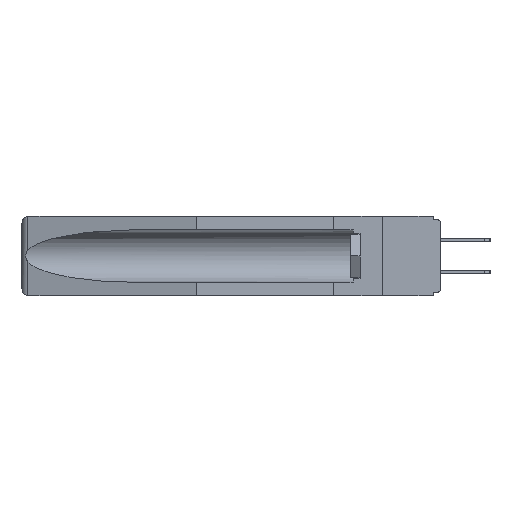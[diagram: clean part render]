
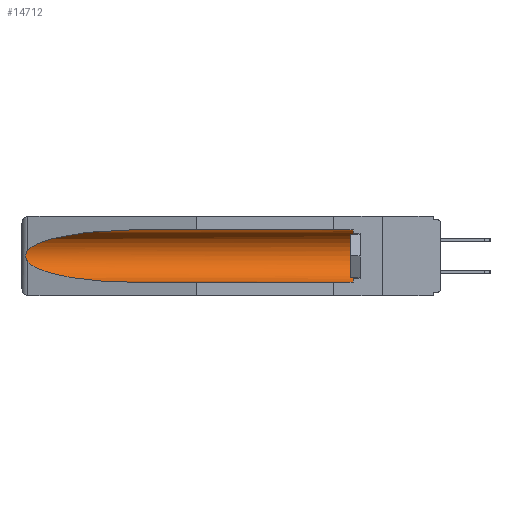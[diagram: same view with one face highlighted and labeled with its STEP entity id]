
A CAD part, left-side view. The second image highlights one B-rep face of the part: STEP entity #14712.
In plain terms, the highlighted cylindrical face has radius 2.857 mm (diameter 5.715 mm), a partial arc.
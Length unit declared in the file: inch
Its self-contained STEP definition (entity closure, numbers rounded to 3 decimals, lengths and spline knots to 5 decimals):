
#1440 = CARTESIAN_POINT ( 'NONE',  ( 0.26654, 1.53092, -0.15636 ) ) ;
#1944 = CARTESIAN_POINT ( 'NONE',  ( 0.155, 0.126, -0.1715 ) ) ;
#2196 = EDGE_CURVE ( 'NONE', #29372, #29384, #31087, .T. ) ;
#2393 = CARTESIAN_POINT ( 'NONE',  ( 0.155, 1.07973, -0.059 ) ) ;
#2695 = LINE ( 'NONE', #21639, #15614 ) ;
#3336 = EDGE_LOOP ( 'NONE', ( #25295, #10266, #11486, #13064, #22401, #14451 ) ) ;
#3780 =( BOUNDED_CURVE ( )  B_SPLINE_CURVE ( 3, ( #4491, #21707, #9361, #7116 ),
 .UNSPECIFIED., .F., .F. ) 
 B_SPLINE_CURVE_WITH_KNOTS ( ( 4, 4 ),
 ( 0.1948, 1.5708 ),
 .UNSPECIFIED. ) 
 CURVE ( )  GEOMETRIC_REPRESENTATION_ITEM ( )  RATIONAL_B_SPLINE_CURVE ( ( 1., 0.848, 0.848, 1. ) ) 
 REPRESENTATION_ITEM ( '' )  );
#3962 = VECTOR ( 'NONE', #27473, 39.37008 ) ;
#4127 = DIRECTION ( 'NONE',  ( 0., 1., 0. ) ) ;
#4421 = CARTESIAN_POINT ( 'NONE',  ( 0.26655, 1.53094, -0.18657 ) ) ;
#4491 = CARTESIAN_POINT ( 'NONE',  ( 0.26537, 1.52718, -0.19328 ) ) ;
#4747 = CARTESIAN_POINT ( 'NONE',  ( 0.2673, 1.53269, -0.17917 ) ) ;
#4952 = CARTESIAN_POINT ( 'NONE',  ( 0.25451, 1.48313, -0.09465 ) ) ;
#6329 = CARTESIAN_POINT ( 'NONE',  ( 0.26537, 1.52718, -0.14972 ) ) ;
#7116 = CARTESIAN_POINT ( 'NONE',  ( 0.155, 1.07973, -0.284 ) ) ;
#7553 = EDGE_CURVE ( 'NONE', #14687, #25336, #3780, .T. ) ;
#8666 = EDGE_CURVE ( 'NONE', #29384, #24623, #2695, .T. ) ;
#9361 = CARTESIAN_POINT ( 'NONE',  ( 0.21114, 1.30732, -0.284 ) ) ;
#9494 = CARTESIAN_POINT ( 'NONE',  ( 0.26537, 1.52718, -0.14972 ) ) ;
#9511 = CARTESIAN_POINT ( 'NONE',  ( 0.2675, 1.53308, -0.17534 ) ) ;
#10046 = LINE ( 'NONE', #15360, #3962 ) ;
#10266 = ORIENTED_EDGE ( 'NONE', *, *, #24511, .T. ) ;
#11486 = ORIENTED_EDGE ( 'NONE', *, *, #7553, .T. ) ;
#11538 = CARTESIAN_POINT ( 'NONE',  ( 0.26537, 1.52718, -0.19328 ) ) ;
#12795 = EDGE_CURVE ( 'NONE', #29372, #25336, #10046, .T. ) ;
#13064 = ORIENTED_EDGE ( 'NONE', *, *, #12795, .F. ) ;
#13914 = AXIS2_PLACEMENT_3D ( 'NONE', #1944, #19039, #16716 ) ;
#14169 = CARTESIAN_POINT ( 'NONE',  ( 0.2675, 1.53308, -0.16763 ) ) ;
#14294 = CARTESIAN_POINT ( 'NONE',  ( 0.155, -0.30754, -0.1715 ) ) ;
#14451 = ORIENTED_EDGE ( 'NONE', *, *, #8666, .T. ) ;
#14687 = VERTEX_POINT ( 'NONE', #11538 ) ;
#14712 = ADVANCED_FACE ( 'NONE', ( #22601 ), #14773, .F. ) ;
#14773 = CYLINDRICAL_SURFACE ( 'NONE', #18576, 0.1125 ) ;
#15360 = CARTESIAN_POINT ( 'NONE',  ( 0.155, -0.30754, -0.284 ) ) ;
#15436 = VERTEX_POINT ( 'NONE', #9494 ) ;
#15614 = VECTOR ( 'NONE', #28836, 39.37008 ) ;
#16200 = CARTESIAN_POINT ( 'NONE',  ( 0.26597, 1.52961, -0.15275 ) ) ;
#16716 = DIRECTION ( 'NONE',  ( 0., 0., 1. ) ) ;
#16719 = CARTESIAN_POINT ( 'NONE',  ( 0.155, 0.126, -0.059 ) ) ;
#18576 = AXIS2_PLACEMENT_3D ( 'NONE', #14294, #4127, #21106 ) ;
#19039 = DIRECTION ( 'NONE',  ( 0., -1., 0. ) ) ;
#19272 = CARTESIAN_POINT ( 'NONE',  ( 0.26537, 1.52718, -0.19328 ) ) ;
#21106 = DIRECTION ( 'NONE',  ( 0., 0., 1. ) ) ;
#21639 = CARTESIAN_POINT ( 'NONE',  ( 0.155, -0.30754, -0.059 ) ) ;
#21707 = CARTESIAN_POINT ( 'NONE',  ( 0.25451, 1.48313, -0.24835 ) ) ;
#22401 = ORIENTED_EDGE ( 'NONE', *, *, #2196, .T. ) ;
#22601 = FACE_OUTER_BOUND ( 'NONE', #3336, .T. ) ;
#24040 = CARTESIAN_POINT ( 'NONE',  ( 0.155, 0.126, -0.284 ) ) ;
#24267 = CARTESIAN_POINT ( 'NONE',  ( 0.21114, 1.30732, -0.059 ) ) ;
#24442 = CARTESIAN_POINT ( 'NONE',  ( 0.155, 1.07973, -0.284 ) ) ;
#24511 = EDGE_CURVE ( 'NONE', #15436, #14687, #24997, .T. ) ;
#24623 = VERTEX_POINT ( 'NONE', #28709 ) ;
#24733 = EDGE_CURVE ( 'NONE', #24623, #15436, #28873, .T. ) ;
#24997 = B_SPLINE_CURVE_WITH_KNOTS ( 'NONE', 3,
 ( #6329, #16200, #1440, #25972, #14169, #9511, #4747, #4421, #28930, #19272 ),
 .UNSPECIFIED., .F., .F.,
 ( 4, 2, 2, 2, 4 ),
 ( 0., 0.00029, 0.00058, 0.00087, 0.00117 ),
 .UNSPECIFIED. ) ;
#25295 = ORIENTED_EDGE ( 'NONE', *, *, #24733, .T. ) ;
#25336 = VERTEX_POINT ( 'NONE', #24442 ) ;
#25972 = CARTESIAN_POINT ( 'NONE',  ( 0.2673, 1.5327, -0.16383 ) ) ;
#27473 = DIRECTION ( 'NONE',  ( 0., 1., 0. ) ) ;
#28709 = CARTESIAN_POINT ( 'NONE',  ( 0.155, 1.07973, -0.059 ) ) ;
#28836 = DIRECTION ( 'NONE',  ( 0., 1., 0. ) ) ;
#28873 =( BOUNDED_CURVE ( )  B_SPLINE_CURVE ( 3, ( #2393, #24267, #4952, #29547 ),
 .UNSPECIFIED., .F., .T. ) 
 B_SPLINE_CURVE_WITH_KNOTS ( ( 4, 4 ),
 ( 4.71239, 6.08839 ),
 .UNSPECIFIED. ) 
 CURVE ( )  GEOMETRIC_REPRESENTATION_ITEM ( )  RATIONAL_B_SPLINE_CURVE ( ( 1., 0.848, 0.848, 1. ) ) 
 REPRESENTATION_ITEM ( '' )  );
#28930 = CARTESIAN_POINT ( 'NONE',  ( 0.26597, 1.5296, -0.19026 ) ) ;
#29372 = VERTEX_POINT ( 'NONE', #24040 ) ;
#29384 = VERTEX_POINT ( 'NONE', #16719 ) ;
#29547 = CARTESIAN_POINT ( 'NONE',  ( 0.26537, 1.52718, -0.14972 ) ) ;
#31087 = CIRCLE ( 'NONE', #13914, 0.1125 ) ;
